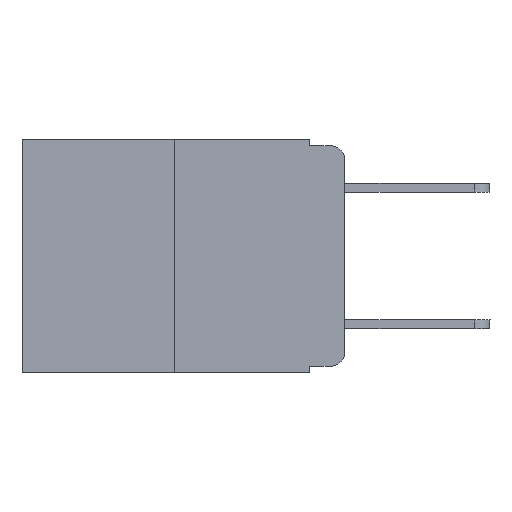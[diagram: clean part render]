
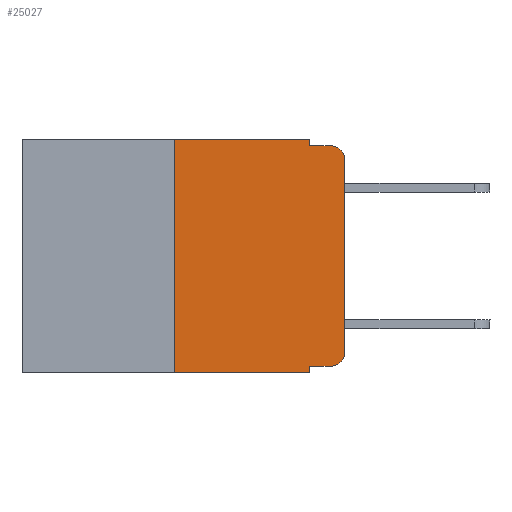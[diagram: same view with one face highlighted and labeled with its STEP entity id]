
A CAD part, left-side view. The second image highlights one B-rep face of the part: STEP entity #25027.
In plain terms, the highlighted planar face has unit normal (-1, 0, 0).
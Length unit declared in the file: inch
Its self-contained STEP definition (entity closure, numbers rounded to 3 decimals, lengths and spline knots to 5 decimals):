
#175 = ORIENTED_EDGE ( 'NONE', *, *, #13085, .F. ) ;
#361 = DIRECTION ( 'NONE',  ( 0., -1., 0. ) ) ;
#636 = CIRCLE ( 'NONE', #15493, 0.02 ) ;
#1197 = LINE ( 'NONE', #7203, #16641 ) ;
#1850 = EDGE_CURVE ( 'NONE', #22207, #16787, #2563, .T. ) ;
#2084 = CARTESIAN_POINT ( 'NONE',  ( 0., 0.051, -0.01 ) ) ;
#2563 = LINE ( 'NONE', #6707, #15670 ) ;
#2799 = VERTEX_POINT ( 'NONE', #15301 ) ;
#2905 = CARTESIAN_POINT ( 'NONE',  ( 0., 0.02, -0.333 ) ) ;
#2925 = CARTESIAN_POINT ( 'NONE',  ( 0., 0.02, -0.01 ) ) ;
#2952 = AXIS2_PLACEMENT_3D ( 'NONE', #11750, #19868, #11881 ) ;
#3517 = CARTESIAN_POINT ( 'NONE',  ( 0., 0.02, -0.03 ) ) ;
#3878 = LINE ( 'NONE', #17706, #8369 ) ;
#3908 = PLANE ( 'NONE',  #2952 ) ;
#3912 = EDGE_LOOP ( 'NONE', ( #7925, #10931, #9786, #175, #8384, #4057, #8054, #14856, #8063, #11891 ) ) ;
#4057 = ORIENTED_EDGE ( 'NONE', *, *, #17831, .F. ) ;
#4150 = VERTEX_POINT ( 'NONE', #18490 ) ;
#4586 = DIRECTION ( 'NONE',  ( 0., 0., 1. ) ) ;
#4905 = CARTESIAN_POINT ( 'NONE',  ( 0., 0.473, -0.343 ) ) ;
#5065 = CARTESIAN_POINT ( 'NONE',  ( 0., 0.051, 0. ) ) ;
#5395 = FACE_OUTER_BOUND ( 'NONE', #3912, .T. ) ;
#5602 = VERTEX_POINT ( 'NONE', #14304 ) ;
#6020 = DIRECTION ( 'NONE',  ( 0., 0., -1. ) ) ;
#6581 = VERTEX_POINT ( 'NONE', #6927 ) ;
#6707 = CARTESIAN_POINT ( 'NONE',  ( 0., 0., 0. ) ) ;
#6847 = LINE ( 'NONE', #8972, #9267 ) ;
#6927 = CARTESIAN_POINT ( 'NONE',  ( 0., 0.051, -0.01 ) ) ;
#7203 = CARTESIAN_POINT ( 'NONE',  ( 0., 0.051, -0.333 ) ) ;
#7254 = VECTOR ( 'NONE', #20824, 39.37008 ) ;
#7260 = CARTESIAN_POINT ( 'NONE',  ( 0., 0.051, -0.343 ) ) ;
#7925 = ORIENTED_EDGE ( 'NONE', *, *, #1850, .T. ) ;
#8054 = ORIENTED_EDGE ( 'NONE', *, *, #23138, .T. ) ;
#8063 = ORIENTED_EDGE ( 'NONE', *, *, #12048, .T. ) ;
#8369 = VECTOR ( 'NONE', #6020, 39.37008 ) ;
#8384 = ORIENTED_EDGE ( 'NONE', *, *, #14716, .F. ) ;
#8397 = VERTEX_POINT ( 'NONE', #2905 ) ;
#8688 = DIRECTION ( 'NONE',  ( -1., 0., 0. ) ) ;
#8733 = CARTESIAN_POINT ( 'NONE',  ( 0., 0., -0.313 ) ) ;
#8776 = VECTOR ( 'NONE', #21523, 39.37008 ) ;
#8807 = AXIS2_PLACEMENT_3D ( 'NONE', #3517, #9911, #17459 ) ;
#8972 = CARTESIAN_POINT ( 'NONE',  ( 0., 0.473, 0. ) ) ;
#9158 = DIRECTION ( 'NONE',  ( 0., -1., 0. ) ) ;
#9267 = VECTOR ( 'NONE', #20670, 39.37008 ) ;
#9699 = VERTEX_POINT ( 'NONE', #7260 ) ;
#9786 = ORIENTED_EDGE ( 'NONE', *, *, #15404, .F. ) ;
#9911 = DIRECTION ( 'NONE',  ( -1., 0., 0. ) ) ;
#10600 = LINE ( 'NONE', #2084, #16978 ) ;
#10931 = ORIENTED_EDGE ( 'NONE', *, *, #23709, .T. ) ;
#11750 = CARTESIAN_POINT ( 'NONE',  ( 0., 0.473, 0. ) ) ;
#11881 = DIRECTION ( 'NONE',  ( 0., 0., -1. ) ) ;
#11891 = ORIENTED_EDGE ( 'NONE', *, *, #19940, .T. ) ;
#12048 = EDGE_CURVE ( 'NONE', #2799, #8397, #1197, .T. ) ;
#12665 = CARTESIAN_POINT ( 'NONE',  ( 0., 0.02, -0.313 ) ) ;
#12727 = CARTESIAN_POINT ( 'NONE',  ( 0., 0.25, 0. ) ) ;
#13085 = EDGE_CURVE ( 'NONE', #4150, #6581, #3878, .T. ) ;
#14304 = CARTESIAN_POINT ( 'NONE',  ( 0., 0.25, 0. ) ) ;
#14716 = EDGE_CURVE ( 'NONE', #5602, #4150, #6847, .T. ) ;
#14856 = ORIENTED_EDGE ( 'NONE', *, *, #22632, .F. ) ;
#15301 = CARTESIAN_POINT ( 'NONE',  ( 0., 0.051, -0.333 ) ) ;
#15404 = EDGE_CURVE ( 'NONE', #6581, #22719, #10600, .T. ) ;
#15493 = AXIS2_PLACEMENT_3D ( 'NONE', #12665, #8688, #20760 ) ;
#15670 = VECTOR ( 'NONE', #4586, 39.37008 ) ;
#16025 = VERTEX_POINT ( 'NONE', #16669 ) ;
#16641 = VECTOR ( 'NONE', #18882, 39.37008 ) ;
#16669 = CARTESIAN_POINT ( 'NONE',  ( 0., 0.25, -0.343 ) ) ;
#16787 = VERTEX_POINT ( 'NONE', #22866 ) ;
#16978 = VECTOR ( 'NONE', #361, 39.37008 ) ;
#17459 = DIRECTION ( 'NONE',  ( 0., 0., -1. ) ) ;
#17670 = VECTOR ( 'NONE', #9158, 39.37008 ) ;
#17706 = CARTESIAN_POINT ( 'NONE',  ( 0., 0.051, 0. ) ) ;
#17831 = EDGE_CURVE ( 'NONE', #16025, #5602, #22279, .T. ) ;
#18490 = CARTESIAN_POINT ( 'NONE',  ( 0., 0.051, 0. ) ) ;
#18882 = DIRECTION ( 'NONE',  ( 0., -1., 0. ) ) ;
#19868 = DIRECTION ( 'NONE',  ( 1., 0., 0. ) ) ;
#19940 = EDGE_CURVE ( 'NONE', #8397, #22207, #636, .T. ) ;
#20246 = CIRCLE ( 'NONE', #8807, 0.02 ) ;
#20670 = DIRECTION ( 'NONE',  ( 0., -1., 0. ) ) ;
#20760 = DIRECTION ( 'NONE',  ( 0., 0., -1. ) ) ;
#20824 = DIRECTION ( 'NONE',  ( 0., 0., 1. ) ) ;
#21129 = LINE ( 'NONE', #5065, #8776 ) ;
#21523 = DIRECTION ( 'NONE',  ( 0., 0., -1. ) ) ;
#22207 = VERTEX_POINT ( 'NONE', #8733 ) ;
#22279 = LINE ( 'NONE', #12727, #7254 ) ;
#22632 = EDGE_CURVE ( 'NONE', #2799, #9699, #21129, .T. ) ;
#22719 = VERTEX_POINT ( 'NONE', #2925 ) ;
#22866 = CARTESIAN_POINT ( 'NONE',  ( 0., 0., -0.03 ) ) ;
#23138 = EDGE_CURVE ( 'NONE', #16025, #9699, #25232, .T. ) ;
#23709 = EDGE_CURVE ( 'NONE', #16787, #22719, #20246, .T. ) ;
#25027 = ADVANCED_FACE ( 'NONE', ( #5395 ), #3908, .F. ) ;
#25232 = LINE ( 'NONE', #4905, #17670 ) ;
